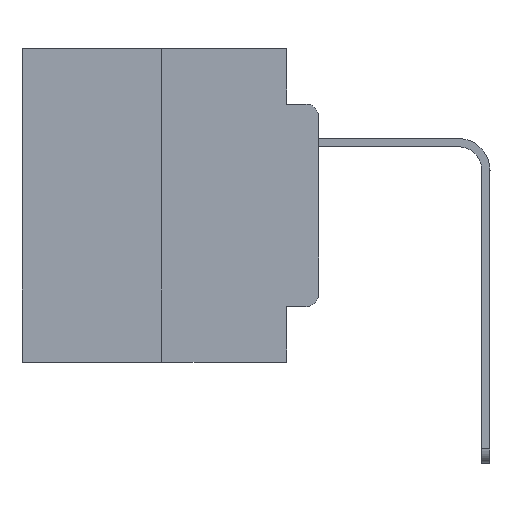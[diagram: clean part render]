
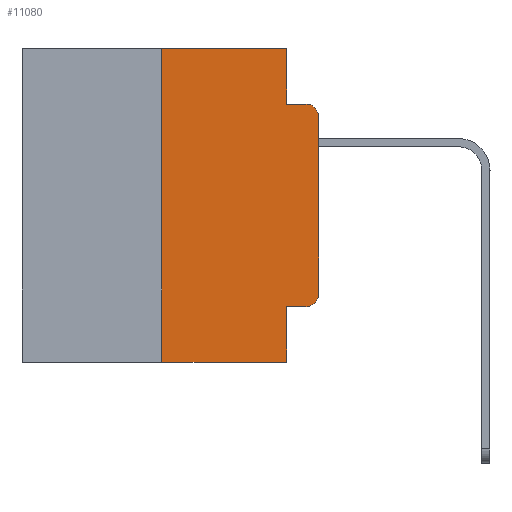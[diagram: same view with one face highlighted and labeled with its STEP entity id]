
A CAD part, left-side view. The second image highlights one B-rep face of the part: STEP entity #11080.
In plain terms, the highlighted planar face has unit normal (-1, 0, 0).
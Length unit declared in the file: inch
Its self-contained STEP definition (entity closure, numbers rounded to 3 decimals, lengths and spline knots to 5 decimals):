
#282 = VECTOR ( 'NONE', #13946, 39.37008 ) ;
#480 = CARTESIAN_POINT ( 'NONE',  ( 0., 0.473, 0. ) ) ;
#562 = DIRECTION ( 'NONE',  ( 0., 0., -1. ) ) ;
#992 = EDGE_CURVE ( 'NONE', #4499, #3564, #26120, .T. ) ;
#1018 = LINE ( 'NONE', #10160, #18481 ) ;
#1499 = DIRECTION ( 'NONE',  ( 0., -1., 0. ) ) ;
#1500 = FACE_OUTER_BOUND ( 'NONE', #5749, .T. ) ;
#1928 = ORIENTED_EDGE ( 'NONE', *, *, #7646, .T. ) ;
#2606 = DIRECTION ( 'NONE',  ( 0., -1., 0. ) ) ;
#2783 = DIRECTION ( 'NONE',  ( -1., 0., 0. ) ) ;
#2867 = CARTESIAN_POINT ( 'NONE',  ( 0., 0.25, 0. ) ) ;
#3203 = CARTESIAN_POINT ( 'NONE',  ( 0., 0.02, -0.0885 ) ) ;
#3497 = VECTOR ( 'NONE', #17502, 39.37008 ) ;
#3564 = VERTEX_POINT ( 'NONE', #24587 ) ;
#3661 = LINE ( 'NONE', #16886, #15427 ) ;
#3723 = EDGE_CURVE ( 'NONE', #25364, #22068, #3661, .T. ) ;
#3884 = DIRECTION ( 'NONE',  ( 0., 0., -1. ) ) ;
#4007 = EDGE_CURVE ( 'NONE', #19943, #17877, #22037, .T. ) ;
#4223 = PLANE ( 'NONE',  #22534 ) ;
#4499 = VERTEX_POINT ( 'NONE', #20411 ) ;
#4735 = EDGE_CURVE ( 'NONE', #3564, #20451, #8732, .T. ) ;
#4814 = AXIS2_PLACEMENT_3D ( 'NONE', #21030, #2783, #12980 ) ;
#5180 = CARTESIAN_POINT ( 'NONE',  ( 0., 0.473, 0. ) ) ;
#5532 = CARTESIAN_POINT ( 'NONE',  ( 0., 0., -0.3915 ) ) ;
#5749 = EDGE_LOOP ( 'NONE', ( #1928, #9555, #11891, #21468, #22515, #22532, #21102, #24065, #25464, #7470 ) ) ;
#7089 = VERTEX_POINT ( 'NONE', #2867 ) ;
#7470 = ORIENTED_EDGE ( 'NONE', *, *, #18143, .T. ) ;
#7646 = EDGE_CURVE ( 'NONE', #19952, #23495, #24219, .T. ) ;
#8668 = AXIS2_PLACEMENT_3D ( 'NONE', #13970, #12183, #14147 ) ;
#8732 = LINE ( 'NONE', #10997, #10307 ) ;
#9401 = CIRCLE ( 'NONE', #4814, 0.02 ) ;
#9555 = ORIENTED_EDGE ( 'NONE', *, *, #16515, .T. ) ;
#10160 = CARTESIAN_POINT ( 'NONE',  ( 0., 0.051, 0. ) ) ;
#10307 = VECTOR ( 'NONE', #19157, 39.37008 ) ;
#10473 = LINE ( 'NONE', #5180, #3497 ) ;
#10997 = CARTESIAN_POINT ( 'NONE',  ( 0., 0.051, -0.0885 ) ) ;
#11080 = ADVANCED_FACE ( 'NONE', ( #1500 ), #4223, .F. ) ;
#11640 = DIRECTION ( 'NONE',  ( 0., 0., 1. ) ) ;
#11891 = ORIENTED_EDGE ( 'NONE', *, *, #4735, .F. ) ;
#11989 = CARTESIAN_POINT ( 'NONE',  ( 0., 0.25, 0. ) ) ;
#12183 = DIRECTION ( 'NONE',  ( -1., 0., 0. ) ) ;
#12980 = DIRECTION ( 'NONE',  ( 0., 0., -1. ) ) ;
#13946 = DIRECTION ( 'NONE',  ( 0., 0., -1. ) ) ;
#13970 = CARTESIAN_POINT ( 'NONE',  ( 0., 0.02, -0.3915 ) ) ;
#14147 = DIRECTION ( 'NONE',  ( 0., 0., -1. ) ) ;
#14249 = EDGE_CURVE ( 'NONE', #7089, #4499, #10473, .T. ) ;
#15124 = CARTESIAN_POINT ( 'NONE',  ( 0., 0.473, -0.5 ) ) ;
#15382 = VECTOR ( 'NONE', #11640, 39.37008 ) ;
#15427 = VECTOR ( 'NONE', #2606, 39.37008 ) ;
#15902 = DIRECTION ( 'NONE',  ( 0., 0., 1. ) ) ;
#16515 = EDGE_CURVE ( 'NONE', #23495, #20451, #9401, .T. ) ;
#16886 = CARTESIAN_POINT ( 'NONE',  ( 0., 0.051, -0.4115 ) ) ;
#17502 = DIRECTION ( 'NONE',  ( 0., -1., 0. ) ) ;
#17690 = CARTESIAN_POINT ( 'NONE',  ( 0., 0.25, -0.5 ) ) ;
#17877 = VERTEX_POINT ( 'NONE', #19207 ) ;
#17902 = CIRCLE ( 'NONE', #8668, 0.02 ) ;
#18143 = EDGE_CURVE ( 'NONE', #22068, #19952, #17902, .T. ) ;
#18481 = VECTOR ( 'NONE', #3884, 39.37008 ) ;
#19157 = DIRECTION ( 'NONE',  ( 0., -1., 0. ) ) ;
#19207 = CARTESIAN_POINT ( 'NONE',  ( 0., 0.051, -0.5 ) ) ;
#19943 = VERTEX_POINT ( 'NONE', #17690 ) ;
#19952 = VERTEX_POINT ( 'NONE', #5532 ) ;
#20411 = CARTESIAN_POINT ( 'NONE',  ( 0., 0.051, 0. ) ) ;
#20451 = VERTEX_POINT ( 'NONE', #3203 ) ;
#21030 = CARTESIAN_POINT ( 'NONE',  ( 0., 0.02, -0.1085 ) ) ;
#21102 = ORIENTED_EDGE ( 'NONE', *, *, #4007, .T. ) ;
#21468 = ORIENTED_EDGE ( 'NONE', *, *, #992, .F. ) ;
#21871 = CARTESIAN_POINT ( 'NONE',  ( 0., 0., -0.1085 ) ) ;
#22037 = LINE ( 'NONE', #15124, #22971 ) ;
#22068 = VERTEX_POINT ( 'NONE', #23186 ) ;
#22172 = CARTESIAN_POINT ( 'NONE',  ( 0., 0.051, -0.4115 ) ) ;
#22515 = ORIENTED_EDGE ( 'NONE', *, *, #14249, .F. ) ;
#22532 = ORIENTED_EDGE ( 'NONE', *, *, #25360, .F. ) ;
#22534 = AXIS2_PLACEMENT_3D ( 'NONE', #480, #24498, #562 ) ;
#22552 = LINE ( 'NONE', #11989, #23497 ) ;
#22971 = VECTOR ( 'NONE', #1499, 39.37008 ) ;
#23186 = CARTESIAN_POINT ( 'NONE',  ( 0., 0.02, -0.4115 ) ) ;
#23495 = VERTEX_POINT ( 'NONE', #21871 ) ;
#23497 = VECTOR ( 'NONE', #15902, 39.37008 ) ;
#23869 = CARTESIAN_POINT ( 'NONE',  ( 0., 0., 0. ) ) ;
#24065 = ORIENTED_EDGE ( 'NONE', *, *, #24826, .F. ) ;
#24219 = LINE ( 'NONE', #23869, #15382 ) ;
#24498 = DIRECTION ( 'NONE',  ( 1., 0., 0. ) ) ;
#24587 = CARTESIAN_POINT ( 'NONE',  ( 0., 0.051, -0.0885 ) ) ;
#24826 = EDGE_CURVE ( 'NONE', #25364, #17877, #1018, .T. ) ;
#25360 = EDGE_CURVE ( 'NONE', #19943, #7089, #22552, .T. ) ;
#25364 = VERTEX_POINT ( 'NONE', #22172 ) ;
#25464 = ORIENTED_EDGE ( 'NONE', *, *, #3723, .T. ) ;
#26047 = CARTESIAN_POINT ( 'NONE',  ( 0., 0.051, 0. ) ) ;
#26120 = LINE ( 'NONE', #26047, #282 ) ;
